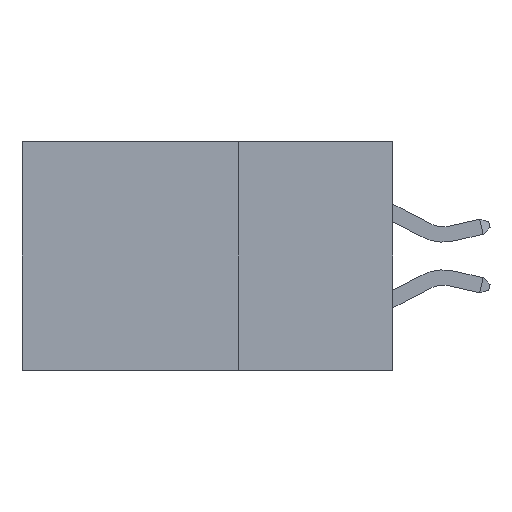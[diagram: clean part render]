
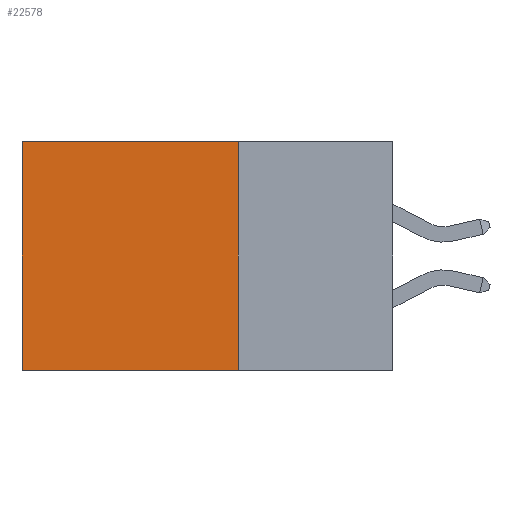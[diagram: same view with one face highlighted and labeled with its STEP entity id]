
A CAD part, left-side view. The second image highlights one B-rep face of the part: STEP entity #22578.
In plain terms, the highlighted planar face has unit normal (-1, 0, 0).
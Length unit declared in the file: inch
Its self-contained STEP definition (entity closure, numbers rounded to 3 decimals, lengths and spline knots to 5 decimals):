
#392 = ORIENTED_EDGE ( 'NONE', *, *, #31287, .F. ) ;
#394 = DIRECTION ( 'NONE',  ( 0., 1., 0. ) ) ;
#1838 = ORIENTED_EDGE ( 'NONE', *, *, #26056, .T. ) ;
#3618 = VECTOR ( 'NONE', #34177, 39.37008 ) ;
#5216 = EDGE_LOOP ( 'NONE', ( #6022, #392, #21544, #1838 ) ) ;
#5895 = CARTESIAN_POINT ( 'NONE',  ( 0.2875, 0.25, 0. ) ) ;
#6022 = ORIENTED_EDGE ( 'NONE', *, *, #21495, .T. ) ;
#7446 = CARTESIAN_POINT ( 'NONE',  ( 0.2875, 0.25, 0. ) ) ;
#8199 = DIRECTION ( 'NONE',  ( 1., 0., 0. ) ) ;
#9464 = LINE ( 'NONE', #23855, #30257 ) ;
#10636 = LINE ( 'NONE', #7446, #3618 ) ;
#11900 = AXIS2_PLACEMENT_3D ( 'NONE', #23691, #8199, #31677 ) ;
#13184 = CARTESIAN_POINT ( 'NONE',  ( 0.2875, 0.6, 0. ) ) ;
#13641 = LINE ( 'NONE', #27884, #22782 ) ;
#13848 = VERTEX_POINT ( 'NONE', #20039 ) ;
#15595 = VERTEX_POINT ( 'NONE', #5895 ) ;
#17693 = DIRECTION ( 'NONE',  ( 0., 1., 0. ) ) ;
#18384 = PLANE ( 'NONE',  #11900 ) ;
#20039 = CARTESIAN_POINT ( 'NONE',  ( 0.2875, 0.6, -0.37 ) ) ;
#21495 = EDGE_CURVE ( 'NONE', #27506, #13848, #13641, .T. ) ;
#21544 = ORIENTED_EDGE ( 'NONE', *, *, #24935, .F. ) ;
#22578 = ADVANCED_FACE ( 'NONE', ( #31489 ), #18384, .F. ) ;
#22782 = VECTOR ( 'NONE', #30568, 39.37008 ) ;
#23691 = CARTESIAN_POINT ( 'NONE',  ( 0.2875, 0.25, 0. ) ) ;
#23855 = CARTESIAN_POINT ( 'NONE',  ( 0.2875, 0.25, -0.37 ) ) ;
#24935 = EDGE_CURVE ( 'NONE', #15595, #33000, #10636, .T. ) ;
#25948 = VECTOR ( 'NONE', #17693, 39.37008 ) ;
#26056 = EDGE_CURVE ( 'NONE', #15595, #27506, #31389, .T. ) ;
#26520 = CARTESIAN_POINT ( 'NONE',  ( 0.2875, 0.25, -0.37 ) ) ;
#27506 = VERTEX_POINT ( 'NONE', #13184 ) ;
#27884 = CARTESIAN_POINT ( 'NONE',  ( 0.2875, 0.6, 0. ) ) ;
#30257 = VECTOR ( 'NONE', #394, 39.37008 ) ;
#30568 = DIRECTION ( 'NONE',  ( 0., 0., -1. ) ) ;
#31287 = EDGE_CURVE ( 'NONE', #33000, #13848, #9464, .T. ) ;
#31389 = LINE ( 'NONE', #34017, #25948 ) ;
#31489 = FACE_OUTER_BOUND ( 'NONE', #5216, .T. ) ;
#31677 = DIRECTION ( 'NONE',  ( 0., 0., -1. ) ) ;
#33000 = VERTEX_POINT ( 'NONE', #26520 ) ;
#34017 = CARTESIAN_POINT ( 'NONE',  ( 0.2875, 0.25, 0. ) ) ;
#34177 = DIRECTION ( 'NONE',  ( 0., 0., -1. ) ) ;
